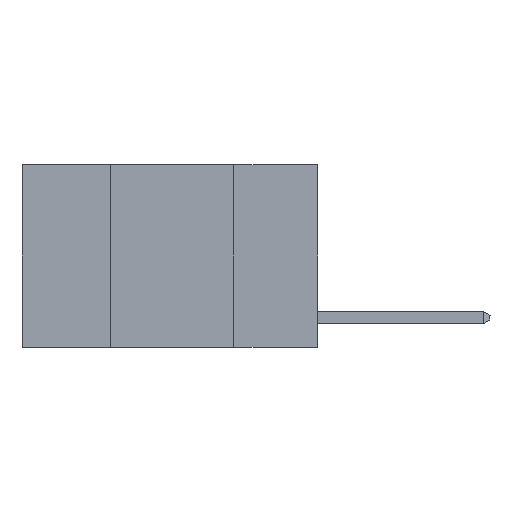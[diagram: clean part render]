
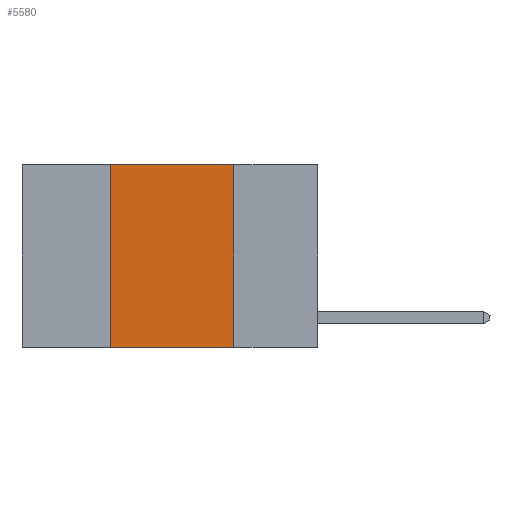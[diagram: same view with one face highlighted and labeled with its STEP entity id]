
A CAD part, left-side view. The second image highlights one B-rep face of the part: STEP entity #5580.
In plain terms, the highlighted planar face has unit normal (-1, 0, 0).
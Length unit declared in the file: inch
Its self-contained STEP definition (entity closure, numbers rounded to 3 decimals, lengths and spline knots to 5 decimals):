
#271 = VERTEX_POINT ( 'NONE', #11796 ) ;
#447 = AXIS2_PLACEMENT_3D ( 'NONE', #14410, #2949, #11155 ) ;
#916 = CARTESIAN_POINT ( 'NONE',  ( 0., 0.42, -0.37 ) ) ;
#1120 = VERTEX_POINT ( 'NONE', #6167 ) ;
#1716 = PLANE ( 'NONE',  #447 ) ;
#1752 = DIRECTION ( 'NONE',  ( 0., 0., -1. ) ) ;
#1776 = ORIENTED_EDGE ( 'NONE', *, *, #6377, .F. ) ;
#1807 = VECTOR ( 'NONE', #11932, 39.37008 ) ;
#2106 = VERTEX_POINT ( 'NONE', #916 ) ;
#2949 = DIRECTION ( 'NONE',  ( 1., 0., 0. ) ) ;
#4113 = ORIENTED_EDGE ( 'NONE', *, *, #10644, .T. ) ;
#4123 = DIRECTION ( 'NONE',  ( 0., 0., 1. ) ) ;
#5580 = ADVANCED_FACE ( 'NONE', ( #11667 ), #1716, .F. ) ;
#5884 = ORIENTED_EDGE ( 'NONE', *, *, #5990, .F. ) ;
#5990 = EDGE_CURVE ( 'NONE', #1120, #271, #10274, .T. ) ;
#6167 = CARTESIAN_POINT ( 'NONE',  ( 0., 0.42, 0. ) ) ;
#6377 = EDGE_CURVE ( 'NONE', #271, #13302, #14678, .T. ) ;
#6750 = EDGE_LOOP ( 'NONE', ( #1776, #5884, #8633, #4113 ) ) ;
#7498 = CARTESIAN_POINT ( 'NONE',  ( 0., 0.17, -0.37 ) ) ;
#8633 = ORIENTED_EDGE ( 'NONE', *, *, #9295, .F. ) ;
#8918 = VECTOR ( 'NONE', #1752, 39.37008 ) ;
#9088 = DIRECTION ( 'NONE',  ( 0., -1., 0. ) ) ;
#9219 = VECTOR ( 'NONE', #4123, 39.37008 ) ;
#9295 = EDGE_CURVE ( 'NONE', #2106, #1120, #12141, .T. ) ;
#9964 = CARTESIAN_POINT ( 'NONE',  ( 0., 0.42, 0. ) ) ;
#10274 = LINE ( 'NONE', #11243, #10601 ) ;
#10601 = VECTOR ( 'NONE', #9088, 39.37008 ) ;
#10644 = EDGE_CURVE ( 'NONE', #2106, #13302, #14128, .T. ) ;
#10786 = CARTESIAN_POINT ( 'NONE',  ( 0., 0.6, -0.37 ) ) ;
#11155 = DIRECTION ( 'NONE',  ( 0., 0., -1. ) ) ;
#11243 = CARTESIAN_POINT ( 'NONE',  ( 0., 0.6, 0. ) ) ;
#11667 = FACE_OUTER_BOUND ( 'NONE', #6750, .T. ) ;
#11796 = CARTESIAN_POINT ( 'NONE',  ( 0., 0.17, 0. ) ) ;
#11932 = DIRECTION ( 'NONE',  ( 0., -1., 0. ) ) ;
#12141 = LINE ( 'NONE', #9964, #9219 ) ;
#12274 = CARTESIAN_POINT ( 'NONE',  ( 0., 0.17, 0. ) ) ;
#13302 = VERTEX_POINT ( 'NONE', #7498 ) ;
#14128 = LINE ( 'NONE', #10786, #1807 ) ;
#14410 = CARTESIAN_POINT ( 'NONE',  ( 0., 0.6, 0. ) ) ;
#14678 = LINE ( 'NONE', #12274, #8918 ) ;
